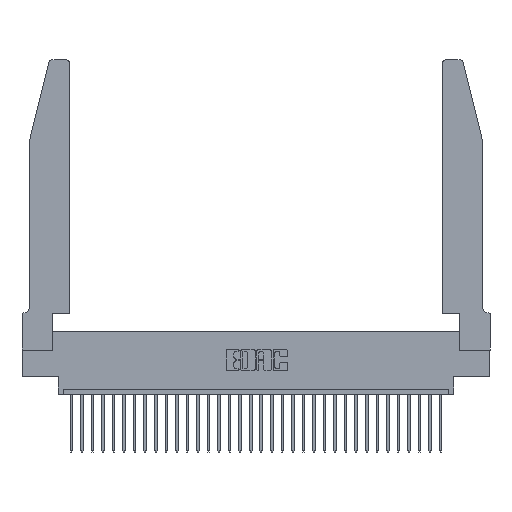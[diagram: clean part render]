
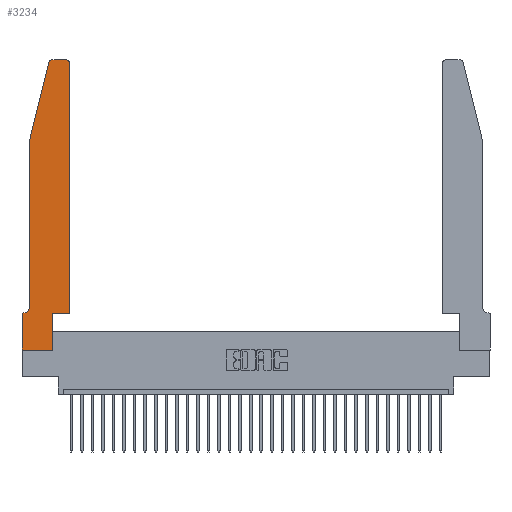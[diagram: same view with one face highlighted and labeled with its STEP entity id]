
A CAD part, top view. The second image highlights one B-rep face of the part: STEP entity #3234.
In plain terms, the highlighted planar face has unit normal (0, 0, 1).
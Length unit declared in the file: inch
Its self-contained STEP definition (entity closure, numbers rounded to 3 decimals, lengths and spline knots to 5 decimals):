
#60 = DIRECTION ( 'NONE',  ( 0., 0., 1. ) ) ;
#124 = CIRCLE ( 'NONE', #768, 0.03 ) ;
#171 = ORIENTED_EDGE ( 'NONE', *, *, #5106, .T. ) ;
#304 = VERTEX_POINT ( 'NONE', #12361 ) ;
#398 = CARTESIAN_POINT ( 'NONE',  ( 0., 0., 0.37 ) ) ;
#620 = EDGE_CURVE ( 'NONE', #21560, #23096, #15127, .T. ) ;
#768 = AXIS2_PLACEMENT_3D ( 'NONE', #21612, #18442, #28023 ) ;
#1127 = EDGE_CURVE ( 'NONE', #11913, #3748, #16279, .T. ) ;
#1559 = CARTESIAN_POINT ( 'NONE',  ( 0.2865, 0.35, 0.37 ) ) ;
#1697 = FACE_OUTER_BOUND ( 'NONE', #8177, .T. ) ;
#2024 = ORIENTED_EDGE ( 'NONE', *, *, #25838, .T. ) ;
#2268 = EDGE_CURVE ( 'NONE', #11530, #304, #23688, .T. ) ;
#2640 = EDGE_CURVE ( 'NONE', #2834, #5958, #19710, .T. ) ;
#2834 = VERTEX_POINT ( 'NONE', #23864 ) ;
#2879 = CIRCLE ( 'NONE', #21165, 0.07 ) ;
#2896 = VERTEX_POINT ( 'NONE', #1559 ) ;
#2902 = DIRECTION ( 'NONE',  ( 1., 0., 0. ) ) ;
#3234 = ADVANCED_FACE ( 'NONE', ( #1697 ), #15112, .T. ) ;
#3256 = VECTOR ( 'NONE', #19840, 39.37008 ) ;
#3748 = VERTEX_POINT ( 'NONE', #18596 ) ;
#5031 = ORIENTED_EDGE ( 'NONE', *, *, #2640, .T. ) ;
#5106 = EDGE_CURVE ( 'NONE', #7977, #2896, #21395, .T. ) ;
#5126 = VECTOR ( 'NONE', #13637, 39.37008 ) ;
#5639 = LINE ( 'NONE', #8942, #7183 ) ;
#5958 = VERTEX_POINT ( 'NONE', #8846 ) ;
#6840 = AXIS2_PLACEMENT_3D ( 'NONE', #29704, #32668, #2902 ) ;
#7183 = VECTOR ( 'NONE', #31529, 39.37008 ) ;
#7245 = ORIENTED_EDGE ( 'NONE', *, *, #24733, .T. ) ;
#7767 = DIRECTION ( 'NONE',  ( 0., -1., 0. ) ) ;
#7977 = VERTEX_POINT ( 'NONE', #24950 ) ;
#8158 = CARTESIAN_POINT ( 'NONE',  ( 0.2605, 2.75, 0.37 ) ) ;
#8177 = EDGE_LOOP ( 'NONE', ( #11325, #5031, #28644, #32050, #22465, #13598, #21587, #32199, #171, #7245, #28657, #2024 ) ) ;
#8471 = CARTESIAN_POINT ( 'NONE',  ( 0.4505, 0.35, 0.37 ) ) ;
#8846 = CARTESIAN_POINT ( 'NONE',  ( 0.25487, 2.72718, 0.37 ) ) ;
#8928 = CARTESIAN_POINT ( 'NONE',  ( 0.4505, 0.35, 0.37 ) ) ;
#8942 = CARTESIAN_POINT ( 'NONE',  ( 0.0755, 0.35, 0.37 ) ) ;
#8955 = LINE ( 'NONE', #8471, #15234 ) ;
#9553 = VECTOR ( 'NONE', #30099, 39.37008 ) ;
#10711 = LINE ( 'NONE', #8158, #17816 ) ;
#11064 = CARTESIAN_POINT ( 'NONE',  ( 0.0055, 0.35, 0.37 ) ) ;
#11325 = ORIENTED_EDGE ( 'NONE', *, *, #14338, .T. ) ;
#11348 = DIRECTION ( 'NONE',  ( 0., 0., -1. ) ) ;
#11530 = VERTEX_POINT ( 'NONE', #8928 ) ;
#11913 = VERTEX_POINT ( 'NONE', #26194 ) ;
#12361 = CARTESIAN_POINT ( 'NONE',  ( 0.4505, 2.72, 0.37 ) ) ;
#13565 = EDGE_CURVE ( 'NONE', #3748, #30609, #2879, .T. ) ;
#13598 = ORIENTED_EDGE ( 'NONE', *, *, #13916, .T. ) ;
#13637 = DIRECTION ( 'NONE',  ( 0., 1., 0. ) ) ;
#13737 = CARTESIAN_POINT ( 'NONE',  ( 0.4505, 0.35, 0.37 ) ) ;
#13916 = EDGE_CURVE ( 'NONE', #30609, #21560, #5639, .T. ) ;
#14338 = EDGE_CURVE ( 'NONE', #30245, #2834, #10711, .T. ) ;
#14443 = CARTESIAN_POINT ( 'NONE',  ( 0.4205, 2.75, 0.37 ) ) ;
#15112 = PLANE ( 'NONE',  #28387 ) ;
#15127 = LINE ( 'NONE', #15492, #18329 ) ;
#15213 = CARTESIAN_POINT ( 'NONE',  ( 0., 0.35, 0.37 ) ) ;
#15234 = VECTOR ( 'NONE', #21033, 39.37008 ) ;
#15296 = VECTOR ( 'NONE', #20630, 39.37008 ) ;
#15492 = CARTESIAN_POINT ( 'NONE',  ( 0., 0., 0.37 ) ) ;
#16279 = LINE ( 'NONE', #19572, #9553 ) ;
#17010 = EDGE_CURVE ( 'NONE', #5958, #11913, #28965, .T. ) ;
#17816 = VECTOR ( 'NONE', #23261, 39.37008 ) ;
#18329 = VECTOR ( 'NONE', #7767, 39.37008 ) ;
#18442 = DIRECTION ( 'NONE',  ( 0., 0., 1. ) ) ;
#18596 = CARTESIAN_POINT ( 'NONE',  ( 0.0755, 0.42, 0.37 ) ) ;
#19196 = DIRECTION ( 'NONE',  ( -0.239, -0.971, 0. ) ) ;
#19572 = CARTESIAN_POINT ( 'NONE',  ( 0.0755, 2., 0.37 ) ) ;
#19710 = CIRCLE ( 'NONE', #6840, 0.03 ) ;
#19840 = DIRECTION ( 'NONE',  ( 0., 1., 0. ) ) ;
#20502 = CARTESIAN_POINT ( 'NONE',  ( 0., 0., 0.37 ) ) ;
#20630 = DIRECTION ( 'NONE',  ( 1., 0., 0. ) ) ;
#21033 = DIRECTION ( 'NONE',  ( 1., 0., 0. ) ) ;
#21165 = AXIS2_PLACEMENT_3D ( 'NONE', #24009, #11348, #26367 ) ;
#21395 = LINE ( 'NONE', #23884, #3256 ) ;
#21397 = DIRECTION ( 'NONE',  ( 1., 0., 0. ) ) ;
#21560 = VERTEX_POINT ( 'NONE', #23989 ) ;
#21587 = ORIENTED_EDGE ( 'NONE', *, *, #620, .T. ) ;
#21612 = CARTESIAN_POINT ( 'NONE',  ( 0.4205, 2.72, 0.37 ) ) ;
#22179 = VECTOR ( 'NONE', #19196, 39.37008 ) ;
#22465 = ORIENTED_EDGE ( 'NONE', *, *, #13565, .T. ) ;
#23096 = VERTEX_POINT ( 'NONE', #20502 ) ;
#23261 = DIRECTION ( 'NONE',  ( -1., 0., 0. ) ) ;
#23688 = LINE ( 'NONE', #13737, #5126 ) ;
#23864 = CARTESIAN_POINT ( 'NONE',  ( 0.284, 2.75, 0.37 ) ) ;
#23884 = CARTESIAN_POINT ( 'NONE',  ( 0.2865, 0.35, 0.37 ) ) ;
#23989 = CARTESIAN_POINT ( 'NONE',  ( 0., 0.35, 0.37 ) ) ;
#24009 = CARTESIAN_POINT ( 'NONE',  ( 0.0055, 0.42, 0.37 ) ) ;
#24045 = EDGE_CURVE ( 'NONE', #23096, #7977, #27152, .T. ) ;
#24733 = EDGE_CURVE ( 'NONE', #2896, #11530, #8955, .T. ) ;
#24950 = CARTESIAN_POINT ( 'NONE',  ( 0.2865, 0., 0.37 ) ) ;
#25838 = EDGE_CURVE ( 'NONE', #304, #30245, #124, .T. ) ;
#26194 = CARTESIAN_POINT ( 'NONE',  ( 0.0755, 2., 0.37 ) ) ;
#26367 = DIRECTION ( 'NONE',  ( -1., 0., 0. ) ) ;
#27152 = LINE ( 'NONE', #398, #15296 ) ;
#28023 = DIRECTION ( 'NONE',  ( 1., 0., 0. ) ) ;
#28387 = AXIS2_PLACEMENT_3D ( 'NONE', #15213, #60, #21397 ) ;
#28644 = ORIENTED_EDGE ( 'NONE', *, *, #17010, .T. ) ;
#28657 = ORIENTED_EDGE ( 'NONE', *, *, #2268, .T. ) ;
#28965 = LINE ( 'NONE', #29814, #22179 ) ;
#29704 = CARTESIAN_POINT ( 'NONE',  ( 0.284, 2.72, 0.37 ) ) ;
#29814 = CARTESIAN_POINT ( 'NONE',  ( 0.0755, 2., 0.37 ) ) ;
#30099 = DIRECTION ( 'NONE',  ( 0., -1., 0. ) ) ;
#30245 = VERTEX_POINT ( 'NONE', #14443 ) ;
#30609 = VERTEX_POINT ( 'NONE', #11064 ) ;
#31529 = DIRECTION ( 'NONE',  ( -1., 0., 0. ) ) ;
#32050 = ORIENTED_EDGE ( 'NONE', *, *, #1127, .T. ) ;
#32199 = ORIENTED_EDGE ( 'NONE', *, *, #24045, .T. ) ;
#32668 = DIRECTION ( 'NONE',  ( 0., 0., 1. ) ) ;
